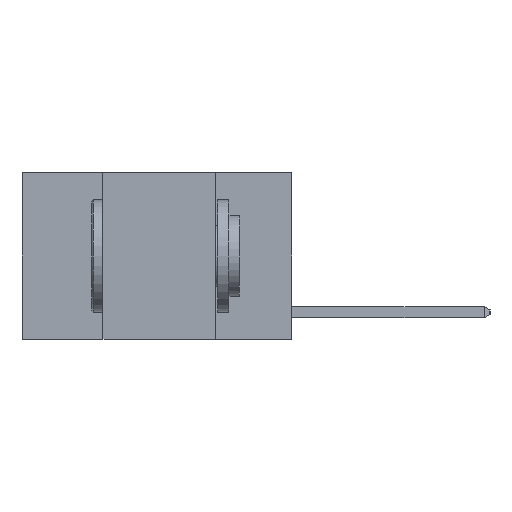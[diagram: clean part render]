
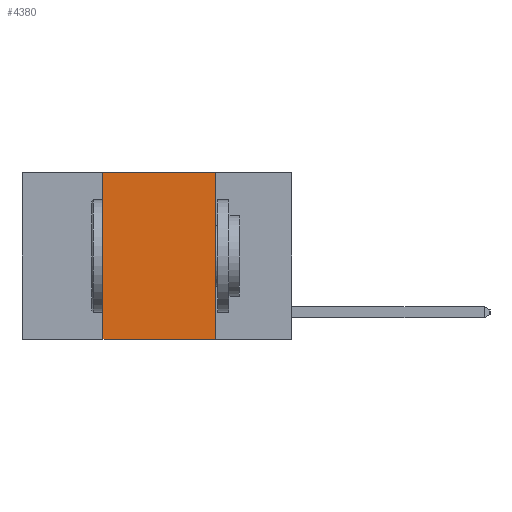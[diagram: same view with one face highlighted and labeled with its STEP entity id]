
A CAD part, left-side view. The second image highlights one B-rep face of the part: STEP entity #4380.
In plain terms, the highlighted planar face has unit normal (-1, 0, 0).
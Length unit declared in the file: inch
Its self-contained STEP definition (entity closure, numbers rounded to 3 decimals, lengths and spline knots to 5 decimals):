
#5 = VECTOR ( 'NONE', #7363, 39.37008 ) ;
#329 = VERTEX_POINT ( 'NONE', #348 ) ;
#348 = CARTESIAN_POINT ( 'NONE',  ( 0., 0.17, 0. ) ) ;
#721 = ORIENTED_EDGE ( 'NONE', *, *, #4754, .F. ) ;
#810 = VERTEX_POINT ( 'NONE', #5019 ) ;
#837 = DIRECTION ( 'NONE',  ( 0., 0., -1. ) ) ;
#1239 = CARTESIAN_POINT ( 'NONE',  ( 0., 0.6, -0.37 ) ) ;
#1447 = VECTOR ( 'NONE', #837, 39.37008 ) ;
#1863 = PLANE ( 'NONE',  #3955 ) ;
#2640 = DIRECTION ( 'NONE',  ( 0., 0., -1. ) ) ;
#2768 = ORIENTED_EDGE ( 'NONE', *, *, #4493, .T. ) ;
#2913 = CARTESIAN_POINT ( 'NONE',  ( 0., 0.42, -0.37 ) ) ;
#3247 = VECTOR ( 'NONE', #6169, 39.37008 ) ;
#3603 = LINE ( 'NONE', #8790, #9403 ) ;
#3611 = LINE ( 'NONE', #1239, #5 ) ;
#3955 = AXIS2_PLACEMENT_3D ( 'NONE', #9434, #7226, #2640 ) ;
#4264 = DIRECTION ( 'NONE',  ( 0., 0., 1. ) ) ;
#4380 = ADVANCED_FACE ( 'NONE', ( #8607 ), #1863, .F. ) ;
#4493 = EDGE_CURVE ( 'NONE', #5143, #8944, #3611, .T. ) ;
#4696 = CARTESIAN_POINT ( 'NONE',  ( 0., 0.17, 0. ) ) ;
#4754 = EDGE_CURVE ( 'NONE', #810, #329, #5528, .T. ) ;
#4991 = EDGE_CURVE ( 'NONE', #5143, #810, #3603, .T. ) ;
#5019 = CARTESIAN_POINT ( 'NONE',  ( 0., 0.42, 0. ) ) ;
#5143 = VERTEX_POINT ( 'NONE', #2913 ) ;
#5393 = CARTESIAN_POINT ( 'NONE',  ( 0., 0.6, 0. ) ) ;
#5524 = ORIENTED_EDGE ( 'NONE', *, *, #4991, .F. ) ;
#5528 = LINE ( 'NONE', #5393, #3247 ) ;
#6015 = EDGE_CURVE ( 'NONE', #329, #8944, #8014, .T. ) ;
#6169 = DIRECTION ( 'NONE',  ( 0., -1., 0. ) ) ;
#6664 = EDGE_LOOP ( 'NONE', ( #7241, #721, #5524, #2768 ) ) ;
#7226 = DIRECTION ( 'NONE',  ( 1., 0., 0. ) ) ;
#7241 = ORIENTED_EDGE ( 'NONE', *, *, #6015, .F. ) ;
#7363 = DIRECTION ( 'NONE',  ( 0., -1., 0. ) ) ;
#7746 = CARTESIAN_POINT ( 'NONE',  ( 0., 0.17, -0.37 ) ) ;
#8014 = LINE ( 'NONE', #4696, #1447 ) ;
#8607 = FACE_OUTER_BOUND ( 'NONE', #6664, .T. ) ;
#8790 = CARTESIAN_POINT ( 'NONE',  ( 0., 0.42, 0. ) ) ;
#8944 = VERTEX_POINT ( 'NONE', #7746 ) ;
#9403 = VECTOR ( 'NONE', #4264, 39.37008 ) ;
#9434 = CARTESIAN_POINT ( 'NONE',  ( 0., 0.6, 0. ) ) ;
